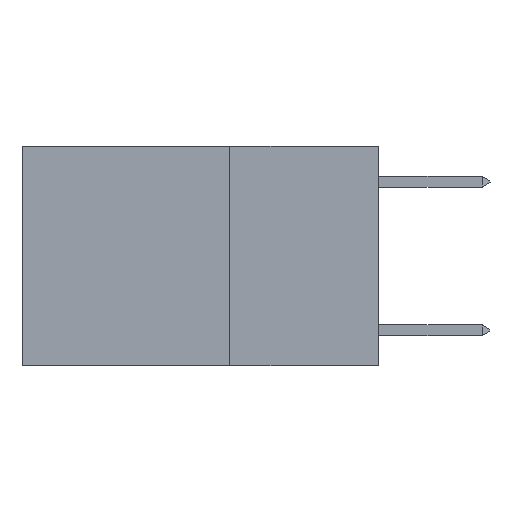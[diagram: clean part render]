
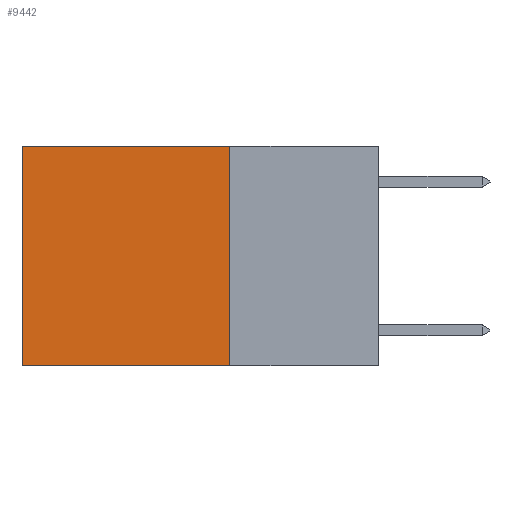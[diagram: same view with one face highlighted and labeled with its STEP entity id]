
A CAD part, left-side view. The second image highlights one B-rep face of the part: STEP entity #9442.
In plain terms, the highlighted planar face has unit normal (-1, 0, 0).
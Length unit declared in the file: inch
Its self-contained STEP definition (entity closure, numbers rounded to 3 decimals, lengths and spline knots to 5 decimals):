
#833 = VECTOR ( 'NONE', #9310, 39.37008 ) ;
#1191 = VERTEX_POINT ( 'NONE', #3473 ) ;
#1442 = AXIS2_PLACEMENT_3D ( 'NONE', #8965, #3154, #2322 ) ;
#1480 = DIRECTION ( 'NONE',  ( 0., 0., -1. ) ) ;
#2322 = DIRECTION ( 'NONE',  ( 0., 0., -1. ) ) ;
#3005 = EDGE_CURVE ( 'NONE', #8280, #6971, #7168, .T. ) ;
#3141 = CARTESIAN_POINT ( 'NONE',  ( 0.2625, 0.25, 0. ) ) ;
#3154 = DIRECTION ( 'NONE',  ( 1., 0., 0. ) ) ;
#3473 = CARTESIAN_POINT ( 'NONE',  ( 0.2625, 0.6, 0. ) ) ;
#3989 = EDGE_LOOP ( 'NONE', ( #8535, #12392, #5163, #5245 ) ) ;
#5021 = CARTESIAN_POINT ( 'NONE',  ( 0.2625, 0.25, 0. ) ) ;
#5163 = ORIENTED_EDGE ( 'NONE', *, *, #3005, .F. ) ;
#5245 = ORIENTED_EDGE ( 'NONE', *, *, #11504, .T. ) ;
#5471 = CARTESIAN_POINT ( 'NONE',  ( 0.2625, 0.6, 0. ) ) ;
#6132 = CARTESIAN_POINT ( 'NONE',  ( 0.2625, 0.25, -0.37 ) ) ;
#6971 = VERTEX_POINT ( 'NONE', #6132 ) ;
#7168 = LINE ( 'NONE', #3141, #7941 ) ;
#7342 = CARTESIAN_POINT ( 'NONE',  ( 0.2625, 0.25, 0. ) ) ;
#7611 = VERTEX_POINT ( 'NONE', #7974 ) ;
#7624 = EDGE_CURVE ( 'NONE', #6971, #7611, #10883, .T. ) ;
#7941 = VECTOR ( 'NONE', #1480, 39.37008 ) ;
#7974 = CARTESIAN_POINT ( 'NONE',  ( 0.2625, 0.6, -0.37 ) ) ;
#8038 = CARTESIAN_POINT ( 'NONE',  ( 0.2625, 0.25, -0.37 ) ) ;
#8280 = VERTEX_POINT ( 'NONE', #7342 ) ;
#8535 = ORIENTED_EDGE ( 'NONE', *, *, #10792, .T. ) ;
#8879 = DIRECTION ( 'NONE',  ( 0., 1., 0. ) ) ;
#8965 = CARTESIAN_POINT ( 'NONE',  ( 0.2625, 0.25, 0. ) ) ;
#9310 = DIRECTION ( 'NONE',  ( 0., 0., -1. ) ) ;
#9442 = ADVANCED_FACE ( 'NONE', ( #9894 ), #10910, .F. ) ;
#9894 = FACE_OUTER_BOUND ( 'NONE', #3989, .T. ) ;
#10258 = LINE ( 'NONE', #5471, #833 ) ;
#10723 = VECTOR ( 'NONE', #11893, 39.37008 ) ;
#10792 = EDGE_CURVE ( 'NONE', #1191, #7611, #10258, .T. ) ;
#10816 = LINE ( 'NONE', #5021, #10853 ) ;
#10853 = VECTOR ( 'NONE', #8879, 39.37008 ) ;
#10883 = LINE ( 'NONE', #8038, #10723 ) ;
#10910 = PLANE ( 'NONE',  #1442 ) ;
#11504 = EDGE_CURVE ( 'NONE', #8280, #1191, #10816, .T. ) ;
#11893 = DIRECTION ( 'NONE',  ( 0., 1., 0. ) ) ;
#12392 = ORIENTED_EDGE ( 'NONE', *, *, #7624, .F. ) ;
